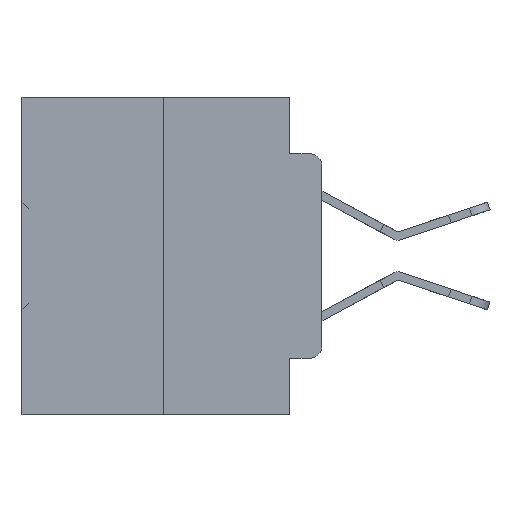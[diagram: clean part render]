
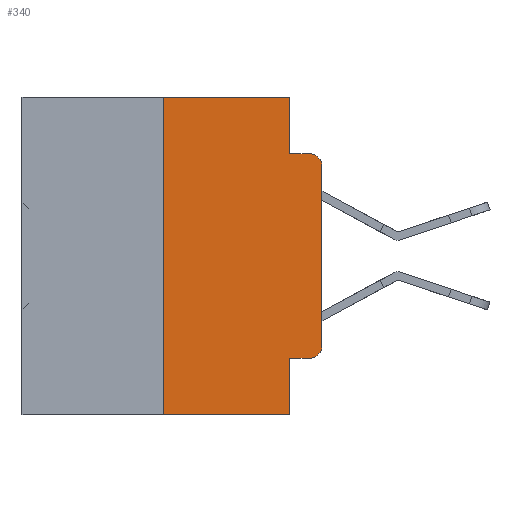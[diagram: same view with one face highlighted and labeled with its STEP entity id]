
A CAD part, left-side view. The second image highlights one B-rep face of the part: STEP entity #340.
In plain terms, the highlighted planar face has unit normal (-1, 0, 0).
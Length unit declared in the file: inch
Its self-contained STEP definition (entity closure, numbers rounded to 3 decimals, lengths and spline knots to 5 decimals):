
#340 = ADVANCED_FACE ( 'NONE', ( #3044 ), #36692, .F. ) ;
#376 = DIRECTION ( 'NONE',  ( 0., -1., 0. ) ) ;
#700 = VERTEX_POINT ( 'NONE', #24635 ) ;
#1527 = EDGE_CURVE ( 'NONE', #38682, #8962, #38256, .T. ) ;
#1984 = DIRECTION ( 'NONE',  ( -1., 0., 0. ) ) ;
#1985 = AXIS2_PLACEMENT_3D ( 'NONE', #34944, #31390, #4724 ) ;
#2276 = VECTOR ( 'NONE', #33286, 39.37008 ) ;
#2894 = LINE ( 'NONE', #23601, #14207 ) ;
#3044 = FACE_OUTER_BOUND ( 'NONE', #8548, .T. ) ;
#3917 = VERTEX_POINT ( 'NONE', #34053 ) ;
#4326 = LINE ( 'NONE', #34987, #11421 ) ;
#4724 = DIRECTION ( 'NONE',  ( 0., 0., -1. ) ) ;
#5014 = DIRECTION ( 'NONE',  ( 0., 0., -1. ) ) ;
#5154 = CARTESIAN_POINT ( 'NONE',  ( 0., 0.02, -0.1085 ) ) ;
#5583 = VECTOR ( 'NONE', #37461, 39.37008 ) ;
#6053 = VERTEX_POINT ( 'NONE', #28906 ) ;
#6171 = VERTEX_POINT ( 'NONE', #8843 ) ;
#6695 = VECTOR ( 'NONE', #31067, 39.37008 ) ;
#6892 = ORIENTED_EDGE ( 'NONE', *, *, #36653, .T. ) ;
#7148 = LINE ( 'NONE', #28040, #6695 ) ;
#7215 = EDGE_CURVE ( 'NONE', #18958, #34009, #7148, .T. ) ;
#8019 = ORIENTED_EDGE ( 'NONE', *, *, #15510, .F. ) ;
#8548 = EDGE_LOOP ( 'NONE', ( #6892, #27065, #32960, #28902, #23899, #8019, #24926, #14409, #24114, #38803 ) ) ;
#8843 = CARTESIAN_POINT ( 'NONE',  ( 0., 0.051, -0.0885 ) ) ;
#8962 = VERTEX_POINT ( 'NONE', #20917 ) ;
#9484 = CIRCLE ( 'NONE', #22283, 0.02 ) ;
#10164 = LINE ( 'NONE', #36366, #32855 ) ;
#10566 = CARTESIAN_POINT ( 'NONE',  ( 0., 0.25, -0.5 ) ) ;
#10576 = DIRECTION ( 'NONE',  ( 0., 0., 1. ) ) ;
#11421 = VECTOR ( 'NONE', #10576, 39.37008 ) ;
#11786 = CARTESIAN_POINT ( 'NONE',  ( 0., 0.02, -0.4115 ) ) ;
#12316 = CARTESIAN_POINT ( 'NONE',  ( 0., 0.051, 0. ) ) ;
#14207 = VECTOR ( 'NONE', #20506, 39.37008 ) ;
#14409 = ORIENTED_EDGE ( 'NONE', *, *, #27970, .F. ) ;
#15510 = EDGE_CURVE ( 'NONE', #18958, #6053, #4326, .T. ) ;
#15588 = DIRECTION ( 'NONE',  ( 1., 0., 0. ) ) ;
#17672 = LINE ( 'NONE', #24178, #34687 ) ;
#18281 = DIRECTION ( 'NONE',  ( 0., -1., 0. ) ) ;
#18781 = EDGE_CURVE ( 'NONE', #6053, #700, #10164, .T. ) ;
#18958 = VERTEX_POINT ( 'NONE', #10566 ) ;
#19434 = VERTEX_POINT ( 'NONE', #39049 ) ;
#20506 = DIRECTION ( 'NONE',  ( 0., 0., -1. ) ) ;
#20917 = CARTESIAN_POINT ( 'NONE',  ( 0., 0., -0.3915 ) ) ;
#21416 = CARTESIAN_POINT ( 'NONE',  ( 0., 0.473, 0. ) ) ;
#22081 = DIRECTION ( 'NONE',  ( 0., -1., 0. ) ) ;
#22283 = AXIS2_PLACEMENT_3D ( 'NONE', #5154, #1984, #5014 ) ;
#22600 = LINE ( 'NONE', #12316, #2276 ) ;
#23601 = CARTESIAN_POINT ( 'NONE',  ( 0., 0.051, 0. ) ) ;
#23899 = ORIENTED_EDGE ( 'NONE', *, *, #18781, .F. ) ;
#24114 = ORIENTED_EDGE ( 'NONE', *, *, #29949, .T. ) ;
#24178 = CARTESIAN_POINT ( 'NONE',  ( 0., 0.051, -0.4115 ) ) ;
#24635 = CARTESIAN_POINT ( 'NONE',  ( 0., 0.051, 0. ) ) ;
#24926 = ORIENTED_EDGE ( 'NONE', *, *, #7215, .T. ) ;
#25311 = CARTESIAN_POINT ( 'NONE',  ( 0., 0.051, -0.5 ) ) ;
#26217 = CARTESIAN_POINT ( 'NONE',  ( 0., 0., -0.1085 ) ) ;
#27065 = ORIENTED_EDGE ( 'NONE', *, *, #34893, .T. ) ;
#27905 = VERTEX_POINT ( 'NONE', #26217 ) ;
#27970 = EDGE_CURVE ( 'NONE', #19434, #34009, #2894, .T. ) ;
#28040 = CARTESIAN_POINT ( 'NONE',  ( 0., 0.473, -0.5 ) ) ;
#28902 = ORIENTED_EDGE ( 'NONE', *, *, #36422, .F. ) ;
#28906 = CARTESIAN_POINT ( 'NONE',  ( 0., 0.25, 0. ) ) ;
#29949 = EDGE_CURVE ( 'NONE', #19434, #38682, #17672, .T. ) ;
#30617 = LINE ( 'NONE', #34189, #5583 ) ;
#30819 = VECTOR ( 'NONE', #22081, 39.37008 ) ;
#31067 = DIRECTION ( 'NONE',  ( 0., -1., 0. ) ) ;
#31390 = DIRECTION ( 'NONE',  ( -1., 0., 0. ) ) ;
#31996 = EDGE_CURVE ( 'NONE', #6171, #3917, #38834, .T. ) ;
#32855 = VECTOR ( 'NONE', #18281, 39.37008 ) ;
#32960 = ORIENTED_EDGE ( 'NONE', *, *, #31996, .F. ) ;
#33286 = DIRECTION ( 'NONE',  ( 0., 0., -1. ) ) ;
#33544 = DIRECTION ( 'NONE',  ( 0., 0., -1. ) ) ;
#33817 = CARTESIAN_POINT ( 'NONE',  ( 0., 0.051, -0.0885 ) ) ;
#34009 = VERTEX_POINT ( 'NONE', #25311 ) ;
#34053 = CARTESIAN_POINT ( 'NONE',  ( 0., 0.02, -0.0885 ) ) ;
#34189 = CARTESIAN_POINT ( 'NONE',  ( 0., 0., 0. ) ) ;
#34687 = VECTOR ( 'NONE', #376, 39.37008 ) ;
#34893 = EDGE_CURVE ( 'NONE', #27905, #3917, #9484, .T. ) ;
#34944 = CARTESIAN_POINT ( 'NONE',  ( 0., 0.02, -0.3915 ) ) ;
#34987 = CARTESIAN_POINT ( 'NONE',  ( 0., 0.25, 0. ) ) ;
#36366 = CARTESIAN_POINT ( 'NONE',  ( 0., 0.473, 0. ) ) ;
#36422 = EDGE_CURVE ( 'NONE', #700, #6171, #22600, .T. ) ;
#36653 = EDGE_CURVE ( 'NONE', #8962, #27905, #30617, .T. ) ;
#36692 = PLANE ( 'NONE',  #38097 ) ;
#37461 = DIRECTION ( 'NONE',  ( 0., 0., 1. ) ) ;
#38097 = AXIS2_PLACEMENT_3D ( 'NONE', #21416, #15588, #33544 ) ;
#38256 = CIRCLE ( 'NONE', #1985, 0.02 ) ;
#38682 = VERTEX_POINT ( 'NONE', #11786 ) ;
#38803 = ORIENTED_EDGE ( 'NONE', *, *, #1527, .T. ) ;
#38834 = LINE ( 'NONE', #33817, #30819 ) ;
#39049 = CARTESIAN_POINT ( 'NONE',  ( 0., 0.051, -0.4115 ) ) ;
